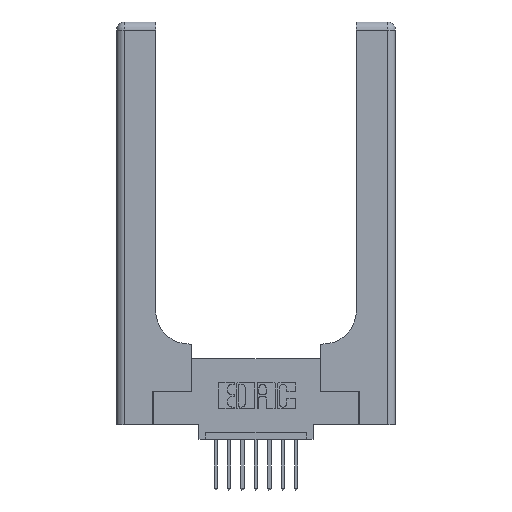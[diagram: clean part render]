
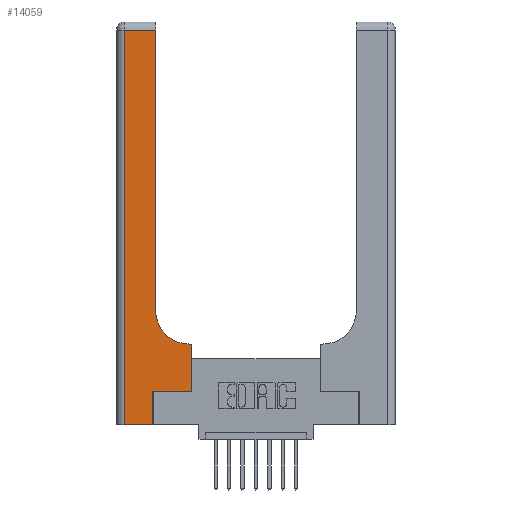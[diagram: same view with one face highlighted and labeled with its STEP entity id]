
A CAD part, top view. The second image highlights one B-rep face of the part: STEP entity #14059.
In plain terms, the highlighted planar face has unit normal (0, 0, 1).
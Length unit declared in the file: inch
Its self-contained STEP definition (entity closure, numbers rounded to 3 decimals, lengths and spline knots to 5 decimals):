
#81 = VERTEX_POINT ( 'NONE', #5504 ) ;
#314 = CARTESIAN_POINT ( 'NONE',  ( 0.5585, 0.6, 0.37 ) ) ;
#321 = CARTESIAN_POINT ( 'NONE',  ( 0.269, 0.25, 0.37 ) ) ;
#342 = CARTESIAN_POINT ( 'NONE',  ( 0.5585, 0.25, 0.37 ) ) ;
#392 = CARTESIAN_POINT ( 'NONE',  ( 0., 3., 0.37 ) ) ;
#406 = DIRECTION ( 'NONE',  ( 1., 0., 0. ) ) ;
#672 = CARTESIAN_POINT ( 'NONE',  ( 0.06, 0., 0.37 ) ) ;
#1383 = FACE_OUTER_BOUND ( 'NONE', #12216, .T. ) ;
#1398 = CARTESIAN_POINT ( 'NONE',  ( 0.5585, 0.25, 0.37 ) ) ;
#1534 = LINE ( 'NONE', #4685, #7613 ) ;
#1789 = DIRECTION ( 'NONE',  ( 0., -1., 0. ) ) ;
#1820 = ORIENTED_EDGE ( 'NONE', *, *, #13595, .T. ) ;
#1970 = LINE ( 'NONE', #12566, #8597 ) ;
#2194 = VECTOR ( 'NONE', #6220, 39.37008 ) ;
#2220 = CIRCLE ( 'NONE', #13020, 0.25 ) ;
#2807 = EDGE_CURVE ( 'NONE', #5168, #14107, #2220, .T. ) ;
#2809 = EDGE_CURVE ( 'NONE', #14107, #81, #2970, .T. ) ;
#2840 = LINE ( 'NONE', #13599, #3397 ) ;
#2970 = LINE ( 'NONE', #4563, #3336 ) ;
#3130 = DIRECTION ( 'NONE',  ( 0., 1., 0. ) ) ;
#3166 = AXIS2_PLACEMENT_3D ( 'NONE', #392, #7548, #7232 ) ;
#3336 = VECTOR ( 'NONE', #7697, 39.37008 ) ;
#3397 = VECTOR ( 'NONE', #5391, 39.37008 ) ;
#3448 = ORIENTED_EDGE ( 'NONE', *, *, #4177, .T. ) ;
#3460 = VERTEX_POINT ( 'NONE', #314 ) ;
#3700 = VERTEX_POINT ( 'NONE', #672 ) ;
#3844 = CARTESIAN_POINT ( 'NONE',  ( 0.2915, 0.6, 0.37 ) ) ;
#4177 = EDGE_CURVE ( 'NONE', #10183, #3460, #7571, .T. ) ;
#4563 = CARTESIAN_POINT ( 'NONE',  ( 0.2915, 3., 0.37 ) ) ;
#4613 = VECTOR ( 'NONE', #1789, 39.37008 ) ;
#4677 = EDGE_CURVE ( 'NONE', #3700, #9590, #6646, .T. ) ;
#4685 = CARTESIAN_POINT ( 'NONE',  ( 0.269, 0.25, 0.37 ) ) ;
#4937 = LINE ( 'NONE', #3844, #7353 ) ;
#5168 = VERTEX_POINT ( 'NONE', #7054 ) ;
#5241 = EDGE_CURVE ( 'NONE', #3460, #5168, #4937, .T. ) ;
#5391 = DIRECTION ( 'NONE',  ( -1., 0., 0. ) ) ;
#5504 = CARTESIAN_POINT ( 'NONE',  ( 0.2915, 2.94, 0.37 ) ) ;
#5693 = CARTESIAN_POINT ( 'NONE',  ( 0.06, 2.94, 0.37 ) ) ;
#5722 = ORIENTED_EDGE ( 'NONE', *, *, #8392, .T. ) ;
#6220 = DIRECTION ( 'NONE',  ( 0., 1., 0. ) ) ;
#6646 = LINE ( 'NONE', #7532, #13464 ) ;
#6724 = ORIENTED_EDGE ( 'NONE', *, *, #14914, .T. ) ;
#6814 = ORIENTED_EDGE ( 'NONE', *, *, #4677, .T. ) ;
#7054 = CARTESIAN_POINT ( 'NONE',  ( 0.5415, 0.6, 0.37 ) ) ;
#7232 = DIRECTION ( 'NONE',  ( -1., 0., 0. ) ) ;
#7353 = VECTOR ( 'NONE', #12094, 39.37008 ) ;
#7494 = PLANE ( 'NONE',  #3166 ) ;
#7532 = CARTESIAN_POINT ( 'NONE',  ( 0., 0., 0.37 ) ) ;
#7548 = DIRECTION ( 'NONE',  ( 0., 0., -1. ) ) ;
#7571 = LINE ( 'NONE', #1398, #2194 ) ;
#7613 = VECTOR ( 'NONE', #11961, 39.37008 ) ;
#7697 = DIRECTION ( 'NONE',  ( 0., 1., 0. ) ) ;
#8392 = EDGE_CURVE ( 'NONE', #10627, #10183, #1534, .T. ) ;
#8597 = VECTOR ( 'NONE', #3130, 39.37008 ) ;
#9361 = ORIENTED_EDGE ( 'NONE', *, *, #2807, .T. ) ;
#9590 = VERTEX_POINT ( 'NONE', #14475 ) ;
#9933 = DIRECTION ( 'NONE',  ( 1., 0., 0. ) ) ;
#9962 = LINE ( 'NONE', #10028, #4613 ) ;
#10028 = CARTESIAN_POINT ( 'NONE',  ( 0.06, 3., 0.37 ) ) ;
#10183 = VERTEX_POINT ( 'NONE', #342 ) ;
#10627 = VERTEX_POINT ( 'NONE', #321 ) ;
#10744 = EDGE_CURVE ( 'NONE', #14367, #3700, #9962, .T. ) ;
#10947 = ORIENTED_EDGE ( 'NONE', *, *, #10744, .T. ) ;
#11032 = CARTESIAN_POINT ( 'NONE',  ( 0.2915, 0.85, 0.37 ) ) ;
#11131 = CARTESIAN_POINT ( 'NONE',  ( 0.5415, 0.85, 0.37 ) ) ;
#11961 = DIRECTION ( 'NONE',  ( 1., 0., 0. ) ) ;
#12016 = ORIENTED_EDGE ( 'NONE', *, *, #5241, .T. ) ;
#12094 = DIRECTION ( 'NONE',  ( -1., 0., 0. ) ) ;
#12216 = EDGE_LOOP ( 'NONE', ( #14533, #6724, #10947, #6814, #1820, #5722, #3448, #12016, #9361 ) ) ;
#12566 = CARTESIAN_POINT ( 'NONE',  ( 0.269, 0., 0.37 ) ) ;
#13020 = AXIS2_PLACEMENT_3D ( 'NONE', #11131, #14713, #406 ) ;
#13464 = VECTOR ( 'NONE', #9933, 39.37008 ) ;
#13595 = EDGE_CURVE ( 'NONE', #9590, #10627, #1970, .T. ) ;
#13599 = CARTESIAN_POINT ( 'NONE',  ( 0., 2.94, 0.37 ) ) ;
#14059 = ADVANCED_FACE ( 'NONE', ( #1383 ), #7494, .F. ) ;
#14107 = VERTEX_POINT ( 'NONE', #11032 ) ;
#14367 = VERTEX_POINT ( 'NONE', #5693 ) ;
#14475 = CARTESIAN_POINT ( 'NONE',  ( 0.269, 0., 0.37 ) ) ;
#14533 = ORIENTED_EDGE ( 'NONE', *, *, #2809, .T. ) ;
#14713 = DIRECTION ( 'NONE',  ( 0., 0., -1. ) ) ;
#14914 = EDGE_CURVE ( 'NONE', #81, #14367, #2840, .T. ) ;
